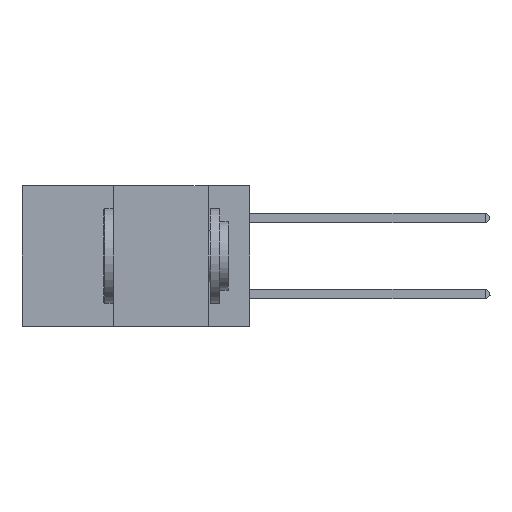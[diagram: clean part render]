
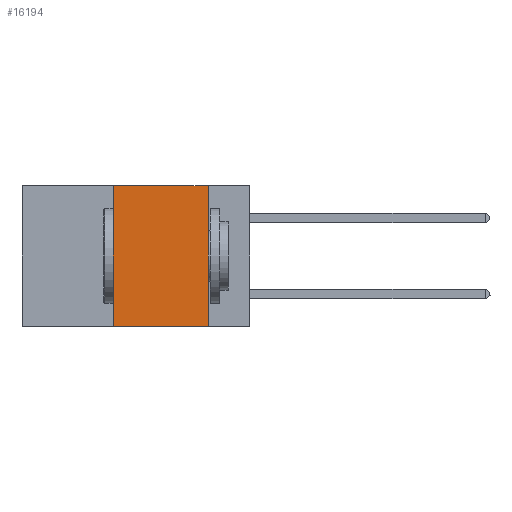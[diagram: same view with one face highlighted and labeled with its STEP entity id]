
A CAD part, left-side view. The second image highlights one B-rep face of the part: STEP entity #16194.
In plain terms, the highlighted planar face has unit normal (-1, 0, 0).
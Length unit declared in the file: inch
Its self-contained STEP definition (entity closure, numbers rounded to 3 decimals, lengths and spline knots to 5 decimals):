
#266 = DIRECTION ( 'NONE',  ( 0., 0., 1. ) ) ;
#389 = CARTESIAN_POINT ( 'NONE',  ( 0., 0.36, 0. ) ) ;
#408 = VECTOR ( 'NONE', #266, 39.37008 ) ;
#475 = VERTEX_POINT ( 'NONE', #15122 ) ;
#639 = CARTESIAN_POINT ( 'NONE',  ( 0., 0.6, 0. ) ) ;
#883 = EDGE_CURVE ( 'NONE', #5140, #475, #11078, .T. ) ;
#1235 = LINE ( 'NONE', #5862, #408 ) ;
#2093 = VECTOR ( 'NONE', #8280, 39.37008 ) ;
#2283 = CARTESIAN_POINT ( 'NONE',  ( 0., 0.11, 0. ) ) ;
#2331 = EDGE_CURVE ( 'NONE', #4017, #475, #16719, .T. ) ;
#2547 = VERTEX_POINT ( 'NONE', #389 ) ;
#3457 = PLANE ( 'NONE',  #15413 ) ;
#3847 = ORIENTED_EDGE ( 'NONE', *, *, #883, .F. ) ;
#4017 = VERTEX_POINT ( 'NONE', #8794 ) ;
#4215 = VECTOR ( 'NONE', #13434, 39.37008 ) ;
#5140 = VERTEX_POINT ( 'NONE', #16489 ) ;
#5408 = ORIENTED_EDGE ( 'NONE', *, *, #2331, .T. ) ;
#5862 = CARTESIAN_POINT ( 'NONE',  ( 0., 0.36, 0. ) ) ;
#6387 = DIRECTION ( 'NONE',  ( 0., 0., -1. ) ) ;
#8280 = DIRECTION ( 'NONE',  ( 0., -1., 0. ) ) ;
#8794 = CARTESIAN_POINT ( 'NONE',  ( 0., 0.36, -0.37 ) ) ;
#9318 = CARTESIAN_POINT ( 'NONE',  ( 0., 0.6, -0.37 ) ) ;
#10109 = DIRECTION ( 'NONE',  ( 0., 0., -1. ) ) ;
#10199 = EDGE_LOOP ( 'NONE', ( #3847, #16640, #16209, #5408 ) ) ;
#11078 = LINE ( 'NONE', #2283, #13990 ) ;
#11185 = CARTESIAN_POINT ( 'NONE',  ( 0., 0.6, 0. ) ) ;
#13115 = FACE_OUTER_BOUND ( 'NONE', #10199, .T. ) ;
#13434 = DIRECTION ( 'NONE',  ( 0., -1., 0. ) ) ;
#13990 = VECTOR ( 'NONE', #6387, 39.37008 ) ;
#15122 = CARTESIAN_POINT ( 'NONE',  ( 0., 0.11, -0.37 ) ) ;
#15413 = AXIS2_PLACEMENT_3D ( 'NONE', #639, #15640, #10109 ) ;
#15640 = DIRECTION ( 'NONE',  ( 1., 0., 0. ) ) ;
#16194 = ADVANCED_FACE ( 'NONE', ( #13115 ), #3457, .F. ) ;
#16209 = ORIENTED_EDGE ( 'NONE', *, *, #16915, .F. ) ;
#16489 = CARTESIAN_POINT ( 'NONE',  ( 0., 0.11, 0. ) ) ;
#16505 = LINE ( 'NONE', #11185, #2093 ) ;
#16640 = ORIENTED_EDGE ( 'NONE', *, *, #16697, .F. ) ;
#16697 = EDGE_CURVE ( 'NONE', #2547, #5140, #16505, .T. ) ;
#16719 = LINE ( 'NONE', #9318, #4215 ) ;
#16915 = EDGE_CURVE ( 'NONE', #4017, #2547, #1235, .T. ) ;
